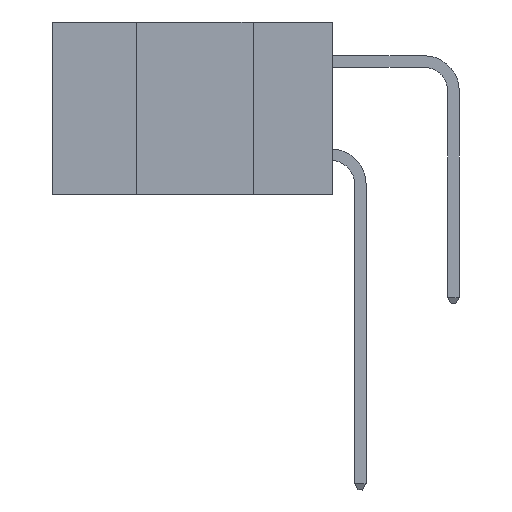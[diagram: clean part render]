
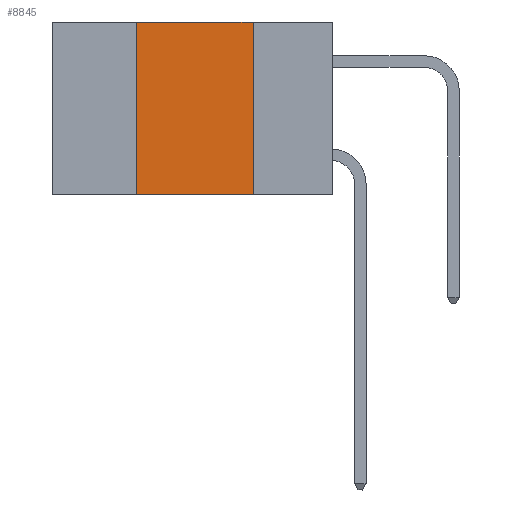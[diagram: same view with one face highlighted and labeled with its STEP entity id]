
A CAD part, left-side view. The second image highlights one B-rep face of the part: STEP entity #8845.
In plain terms, the highlighted planar face has unit normal (-1, 0, 0).
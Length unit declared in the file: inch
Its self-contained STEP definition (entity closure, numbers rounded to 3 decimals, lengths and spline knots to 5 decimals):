
#623 = VECTOR ( 'NONE', #7630, 39.37008 ) ;
#1599 = CARTESIAN_POINT ( 'NONE',  ( 0., 0.17, -0.37 ) ) ;
#2341 = VERTEX_POINT ( 'NONE', #12864 ) ;
#2805 = LINE ( 'NONE', #6837, #5994 ) ;
#2999 = AXIS2_PLACEMENT_3D ( 'NONE', #4185, #4434, #10747 ) ;
#3750 = CARTESIAN_POINT ( 'NONE',  ( 0., 0.6, -0.37 ) ) ;
#4070 = FACE_OUTER_BOUND ( 'NONE', #10321, .T. ) ;
#4144 = DIRECTION ( 'NONE',  ( 0., 0., 1. ) ) ;
#4185 = CARTESIAN_POINT ( 'NONE',  ( 0., 0.6, 0. ) ) ;
#4434 = DIRECTION ( 'NONE',  ( 1., 0., 0. ) ) ;
#4583 = VECTOR ( 'NONE', #5485, 39.37008 ) ;
#4701 = ORIENTED_EDGE ( 'NONE', *, *, #11090, .F. ) ;
#5485 = DIRECTION ( 'NONE',  ( 0., 0., -1. ) ) ;
#5994 = VECTOR ( 'NONE', #4144, 39.37008 ) ;
#6110 = ORIENTED_EDGE ( 'NONE', *, *, #6270, .F. ) ;
#6270 = EDGE_CURVE ( 'NONE', #11382, #8156, #6740, .T. ) ;
#6740 = LINE ( 'NONE', #11870, #4583 ) ;
#6837 = CARTESIAN_POINT ( 'NONE',  ( 0., 0.42, -0.37 ) ) ;
#7630 = DIRECTION ( 'NONE',  ( 0., -1., 0. ) ) ;
#8156 = VERTEX_POINT ( 'NONE', #1599 ) ;
#8845 = ADVANCED_FACE ( 'NONE', ( #4070 ), #9211, .F. ) ;
#8966 = LINE ( 'NONE', #3750, #623 ) ;
#9211 = PLANE ( 'NONE',  #2999 ) ;
#9952 = CARTESIAN_POINT ( 'NONE',  ( 0., 0.6, 0. ) ) ;
#10186 = CARTESIAN_POINT ( 'NONE',  ( 0., 0.17, 0. ) ) ;
#10321 = EDGE_LOOP ( 'NONE', ( #6110, #15994, #4701, #13935 ) ) ;
#10552 = EDGE_CURVE ( 'NONE', #12260, #8156, #8966, .T. ) ;
#10747 = DIRECTION ( 'NONE',  ( 0., 0., -1. ) ) ;
#11090 = EDGE_CURVE ( 'NONE', #12260, #2341, #2805, .T. ) ;
#11382 = VERTEX_POINT ( 'NONE', #10186 ) ;
#11870 = CARTESIAN_POINT ( 'NONE',  ( 0., 0.17, -0.37 ) ) ;
#12157 = EDGE_CURVE ( 'NONE', #2341, #11382, #14853, .T. ) ;
#12260 = VERTEX_POINT ( 'NONE', #13579 ) ;
#12864 = CARTESIAN_POINT ( 'NONE',  ( 0., 0.42, 0. ) ) ;
#13579 = CARTESIAN_POINT ( 'NONE',  ( 0., 0.42, -0.37 ) ) ;
#13935 = ORIENTED_EDGE ( 'NONE', *, *, #10552, .T. ) ;
#14625 = VECTOR ( 'NONE', #16120, 39.37008 ) ;
#14853 = LINE ( 'NONE', #9952, #14625 ) ;
#15994 = ORIENTED_EDGE ( 'NONE', *, *, #12157, .F. ) ;
#16120 = DIRECTION ( 'NONE',  ( 0., -1., 0. ) ) ;
